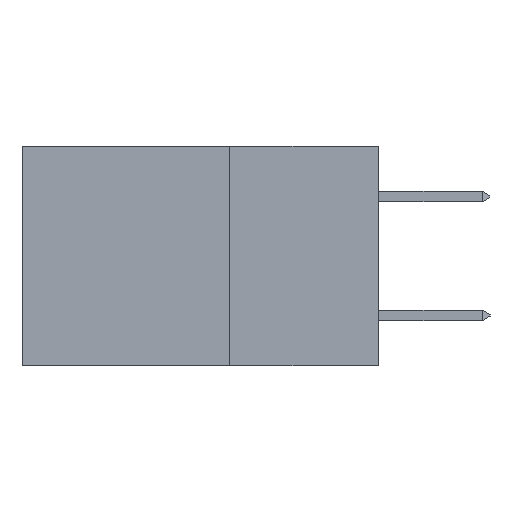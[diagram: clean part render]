
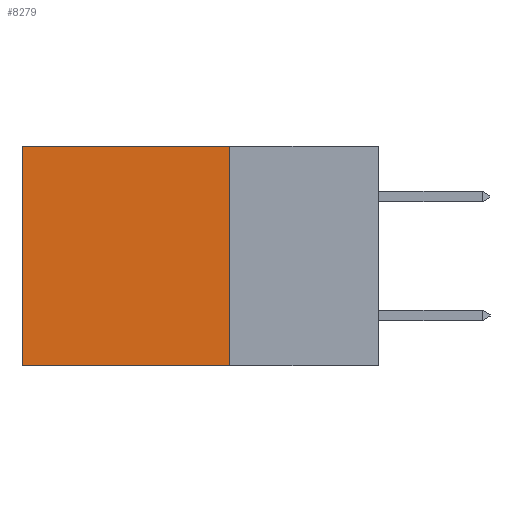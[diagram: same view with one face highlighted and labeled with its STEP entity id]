
A CAD part, left-side view. The second image highlights one B-rep face of the part: STEP entity #8279.
In plain terms, the highlighted planar face has unit normal (-1, 0, 0).
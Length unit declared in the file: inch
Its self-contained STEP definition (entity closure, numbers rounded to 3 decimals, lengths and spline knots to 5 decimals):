
#196 = VERTEX_POINT ( 'NONE', #13468 ) ;
#981 = ORIENTED_EDGE ( 'NONE', *, *, #11081, .T. ) ;
#1178 = CARTESIAN_POINT ( 'NONE',  ( 0.2615, 0.6, -0.37 ) ) ;
#1464 = DIRECTION ( 'NONE',  ( 0., 0., -1. ) ) ;
#2179 = CARTESIAN_POINT ( 'NONE',  ( 0.2615, 0.25, 0. ) ) ;
#2444 = VECTOR ( 'NONE', #15509, 39.37008 ) ;
#3455 = ORIENTED_EDGE ( 'NONE', *, *, #13541, .T. ) ;
#5193 = AXIS2_PLACEMENT_3D ( 'NONE', #16840, #14309, #6371 ) ;
#5429 = ORIENTED_EDGE ( 'NONE', *, *, #14754, .F. ) ;
#5577 = ORIENTED_EDGE ( 'NONE', *, *, #9463, .F. ) ;
#5793 = LINE ( 'NONE', #5988, #6221 ) ;
#5988 = CARTESIAN_POINT ( 'NONE',  ( 0.2615, 0.25, -0.37 ) ) ;
#6221 = VECTOR ( 'NONE', #12616, 39.37008 ) ;
#6371 = DIRECTION ( 'NONE',  ( 0., 0., -1. ) ) ;
#6569 = VERTEX_POINT ( 'NONE', #1178 ) ;
#7605 = VECTOR ( 'NONE', #15261, 39.37008 ) ;
#8279 = ADVANCED_FACE ( 'NONE', ( #16953 ), #11635, .F. ) ;
#9463 = EDGE_CURVE ( 'NONE', #13433, #12030, #5793, .T. ) ;
#11081 = EDGE_CURVE ( 'NONE', #196, #6569, #16263, .T. ) ;
#11118 = LINE ( 'NONE', #11221, #7605 ) ;
#11221 = CARTESIAN_POINT ( 'NONE',  ( 0.2615, 0.25, -0.37 ) ) ;
#11635 = PLANE ( 'NONE',  #5193 ) ;
#12030 = VERTEX_POINT ( 'NONE', #15288 ) ;
#12160 = EDGE_LOOP ( 'NONE', ( #981, #5429, #5577, #3455 ) ) ;
#12616 = DIRECTION ( 'NONE',  ( 0., 0., -1. ) ) ;
#12851 = VECTOR ( 'NONE', #1464, 39.37008 ) ;
#13433 = VERTEX_POINT ( 'NONE', #16785 ) ;
#13468 = CARTESIAN_POINT ( 'NONE',  ( 0.2615, 0.6, 0. ) ) ;
#13541 = EDGE_CURVE ( 'NONE', #13433, #196, #16510, .T. ) ;
#14309 = DIRECTION ( 'NONE',  ( 1., 0., 0. ) ) ;
#14747 = CARTESIAN_POINT ( 'NONE',  ( 0.2615, 0.6, -0.37 ) ) ;
#14754 = EDGE_CURVE ( 'NONE', #12030, #6569, #11118, .T. ) ;
#15261 = DIRECTION ( 'NONE',  ( 0., 1., 0. ) ) ;
#15288 = CARTESIAN_POINT ( 'NONE',  ( 0.2615, 0.25, -0.37 ) ) ;
#15509 = DIRECTION ( 'NONE',  ( 0., 1., 0. ) ) ;
#16263 = LINE ( 'NONE', #14747, #12851 ) ;
#16510 = LINE ( 'NONE', #2179, #2444 ) ;
#16785 = CARTESIAN_POINT ( 'NONE',  ( 0.2615, 0.25, 0. ) ) ;
#16840 = CARTESIAN_POINT ( 'NONE',  ( 0.2615, 0.25, -0.37 ) ) ;
#16953 = FACE_OUTER_BOUND ( 'NONE', #12160, .T. ) ;
